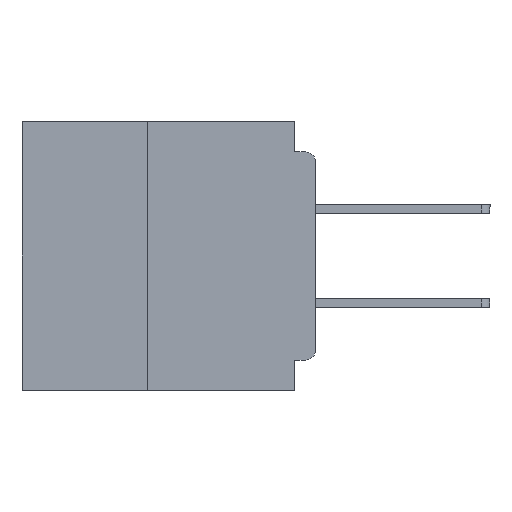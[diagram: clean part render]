
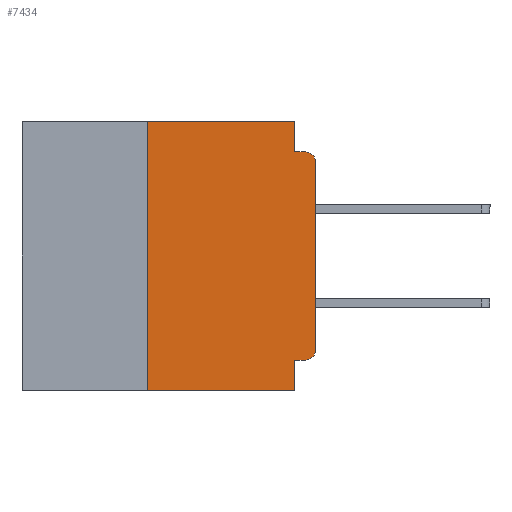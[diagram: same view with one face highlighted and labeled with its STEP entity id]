
A CAD part, left-side view. The second image highlights one B-rep face of the part: STEP entity #7434.
In plain terms, the highlighted planar face has unit normal (-1, 0, 0).
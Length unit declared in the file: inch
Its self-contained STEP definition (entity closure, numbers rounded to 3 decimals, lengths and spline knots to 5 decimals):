
#218 = CARTESIAN_POINT ( 'NONE',  ( 0., 0.25, -0.4 ) ) ;
#2009 = DIRECTION ( 'NONE',  ( 0., 1., 0. ) ) ;
#2163 = LINE ( 'NONE', #18558, #29936 ) ;
#2246 = LINE ( 'NONE', #35869, #33859 ) ;
#2310 = VERTEX_POINT ( 'NONE', #50450 ) ;
#2313 = EDGE_CURVE ( 'NONE', #25070, #42188, #50688, .T. ) ;
#2904 = DIRECTION ( 'NONE',  ( 1., 0., 0. ) ) ;
#3108 = CARTESIAN_POINT ( 'NONE',  ( 0., 0.031, -0.355 ) ) ;
#3940 = CARTESIAN_POINT ( 'NONE',  ( 0., 0.031, -0.4 ) ) ;
#5452 = CARTESIAN_POINT ( 'NONE',  ( 0., 0.031, 0. ) ) ;
#5652 = EDGE_LOOP ( 'NONE', ( #19032, #17309, #10237, #35725, #16531, #40081, #23244, #27121, #14771, #34072 ) ) ;
#5665 = VERTEX_POINT ( 'NONE', #11712 ) ;
#5739 = LINE ( 'NONE', #31492, #27750 ) ;
#7434 = ADVANCED_FACE ( 'NONE', ( #50711 ), #47871, .F. ) ;
#8344 = DIRECTION ( 'NONE',  ( 0., 0., -1. ) ) ;
#8904 = VECTOR ( 'NONE', #2009, 39.37008 ) ;
#9519 = CARTESIAN_POINT ( 'NONE',  ( 0., 0., -0.34 ) ) ;
#9767 = EDGE_CURVE ( 'NONE', #22531, #5665, #36738, .T. ) ;
#10237 = ORIENTED_EDGE ( 'NONE', *, *, #49044, .F. ) ;
#11135 = DIRECTION ( 'NONE',  ( -1., 0., 0. ) ) ;
#11712 = CARTESIAN_POINT ( 'NONE',  ( 0., 0.031, -0.045 ) ) ;
#12256 = AXIS2_PLACEMENT_3D ( 'NONE', #51861, #2904, #31797 ) ;
#12524 = CARTESIAN_POINT ( 'NONE',  ( 0., 0.031, -0.4 ) ) ;
#14551 = DIRECTION ( 'NONE',  ( 0., 0., 1. ) ) ;
#14571 = CARTESIAN_POINT ( 'NONE',  ( 0., 0.437, -0.4 ) ) ;
#14771 = ORIENTED_EDGE ( 'NONE', *, *, #50191, .F. ) ;
#14845 = VERTEX_POINT ( 'NONE', #31034 ) ;
#16069 = VECTOR ( 'NONE', #30232, 39.37008 ) ;
#16531 = ORIENTED_EDGE ( 'NONE', *, *, #24285, .F. ) ;
#16865 = EDGE_CURVE ( 'NONE', #42188, #26748, #2163, .T. ) ;
#17309 = ORIENTED_EDGE ( 'NONE', *, *, #24234, .T. ) ;
#17365 = EDGE_CURVE ( 'NONE', #19753, #43892, #28601, .T. ) ;
#17688 = VECTOR ( 'NONE', #44336, 39.37008 ) ;
#18558 = CARTESIAN_POINT ( 'NONE',  ( 0., 0., 0. ) ) ;
#19032 = ORIENTED_EDGE ( 'NONE', *, *, #16865, .T. ) ;
#19753 = VERTEX_POINT ( 'NONE', #3108 ) ;
#19848 = CARTESIAN_POINT ( 'NONE',  ( 0., 0.437, 0. ) ) ;
#22531 = VERTEX_POINT ( 'NONE', #46455 ) ;
#22821 = VECTOR ( 'NONE', #51308, 39.37008 ) ;
#23244 = ORIENTED_EDGE ( 'NONE', *, *, #42359, .T. ) ;
#24131 = LINE ( 'NONE', #14571, #22821 ) ;
#24234 = EDGE_CURVE ( 'NONE', #26748, #2310, #42087, .T. ) ;
#24285 = EDGE_CURVE ( 'NONE', #14845, #22531, #39569, .T. ) ;
#25070 = VERTEX_POINT ( 'NONE', #49141 ) ;
#26748 = VERTEX_POINT ( 'NONE', #36868 ) ;
#27121 = ORIENTED_EDGE ( 'NONE', *, *, #17365, .F. ) ;
#27750 = VECTOR ( 'NONE', #51583, 39.37008 ) ;
#28601 = LINE ( 'NONE', #12524, #38146 ) ;
#29027 = AXIS2_PLACEMENT_3D ( 'NONE', #48629, #48512, #48396 ) ;
#29936 = VECTOR ( 'NONE', #14551, 39.37008 ) ;
#30232 = DIRECTION ( 'NONE',  ( 0., 0., -1. ) ) ;
#30326 = VERTEX_POINT ( 'NONE', #218 ) ;
#31034 = CARTESIAN_POINT ( 'NONE',  ( 0., 0.25, 0. ) ) ;
#31492 = CARTESIAN_POINT ( 'NONE',  ( 0., 0.25, -0.4 ) ) ;
#31797 = DIRECTION ( 'NONE',  ( 0., 0., -1. ) ) ;
#33859 = VECTOR ( 'NONE', #51976, 39.37008 ) ;
#34072 = ORIENTED_EDGE ( 'NONE', *, *, #2313, .T. ) ;
#35725 = ORIENTED_EDGE ( 'NONE', *, *, #9767, .F. ) ;
#35869 = CARTESIAN_POINT ( 'NONE',  ( 0., 0., -0.045 ) ) ;
#35876 = CARTESIAN_POINT ( 'NONE',  ( 0., 0.015, -0.06 ) ) ;
#36738 = LINE ( 'NONE', #5452, #16069 ) ;
#36868 = CARTESIAN_POINT ( 'NONE',  ( 0., 0., -0.06 ) ) ;
#38146 = VECTOR ( 'NONE', #8344, 39.37008 ) ;
#39569 = LINE ( 'NONE', #19848, #17688 ) ;
#39942 = DIRECTION ( 'NONE',  ( 0., 0., -1. ) ) ;
#40081 = ORIENTED_EDGE ( 'NONE', *, *, #49656, .F. ) ;
#40485 = LINE ( 'NONE', #51015, #8904 ) ;
#42087 = CIRCLE ( 'NONE', #45710, 0.015 ) ;
#42188 = VERTEX_POINT ( 'NONE', #9519 ) ;
#42359 = EDGE_CURVE ( 'NONE', #30326, #43892, #24131, .T. ) ;
#43892 = VERTEX_POINT ( 'NONE', #3940 ) ;
#44336 = DIRECTION ( 'NONE',  ( 0., -1., 0. ) ) ;
#45710 = AXIS2_PLACEMENT_3D ( 'NONE', #35876, #11135, #39942 ) ;
#46455 = CARTESIAN_POINT ( 'NONE',  ( 0., 0.031, 0. ) ) ;
#47871 = PLANE ( 'NONE',  #12256 ) ;
#48396 = DIRECTION ( 'NONE',  ( 0., 0., -1. ) ) ;
#48512 = DIRECTION ( 'NONE',  ( -1., 0., 0. ) ) ;
#48629 = CARTESIAN_POINT ( 'NONE',  ( 0., 0.015, -0.34 ) ) ;
#49044 = EDGE_CURVE ( 'NONE', #5665, #2310, #2246, .T. ) ;
#49141 = CARTESIAN_POINT ( 'NONE',  ( 0., 0.015, -0.355 ) ) ;
#49656 = EDGE_CURVE ( 'NONE', #30326, #14845, #5739, .T. ) ;
#50191 = EDGE_CURVE ( 'NONE', #25070, #19753, #40485, .T. ) ;
#50450 = CARTESIAN_POINT ( 'NONE',  ( 0., 0.015, -0.045 ) ) ;
#50688 = CIRCLE ( 'NONE', #29027, 0.015 ) ;
#50711 = FACE_OUTER_BOUND ( 'NONE', #5652, .T. ) ;
#51015 = CARTESIAN_POINT ( 'NONE',  ( 0., 0., -0.355 ) ) ;
#51308 = DIRECTION ( 'NONE',  ( 0., -1., 0. ) ) ;
#51583 = DIRECTION ( 'NONE',  ( 0., 0., 1. ) ) ;
#51861 = CARTESIAN_POINT ( 'NONE',  ( 0., 0.437, 0. ) ) ;
#51976 = DIRECTION ( 'NONE',  ( 0., -1., 0. ) ) ;
